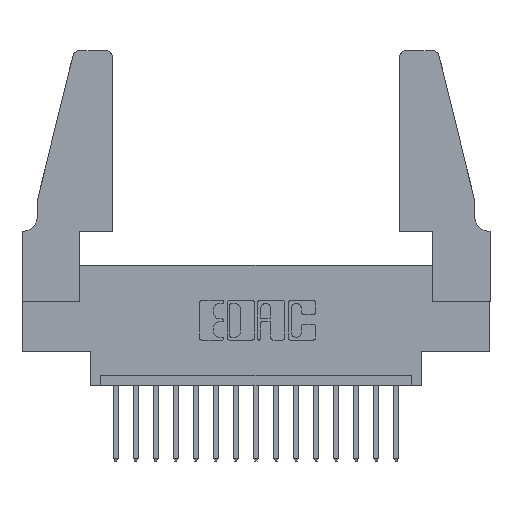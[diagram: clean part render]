
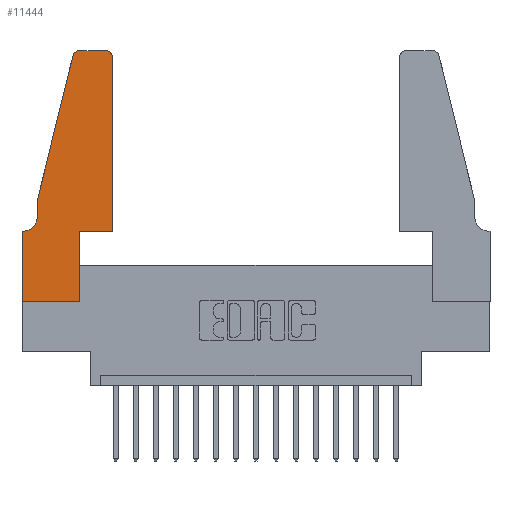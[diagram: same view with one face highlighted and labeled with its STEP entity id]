
A CAD part, top view. The second image highlights one B-rep face of the part: STEP entity #11444.
In plain terms, the highlighted planar face has unit normal (0, 0, 1).
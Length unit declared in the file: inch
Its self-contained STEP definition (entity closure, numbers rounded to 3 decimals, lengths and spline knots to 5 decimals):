
#1 = ORIENTED_EDGE ( 'NONE', *, *, #2793, .T. ) ;
#16 = VERTEX_POINT ( 'NONE', #2848 ) ;
#237 = VERTEX_POINT ( 'NONE', #4636 ) ;
#336 = CARTESIAN_POINT ( 'NONE',  ( 0.2865, 0.35, 0.37 ) ) ;
#346 = CARTESIAN_POINT ( 'NONE',  ( 0., 0.35, 0.37 ) ) ;
#474 = CARTESIAN_POINT ( 'NONE',  ( 0.284, 1.22, 0.37 ) ) ;
#496 = LINE ( 'NONE', #1769, #7144 ) ;
#559 = CIRCLE ( 'NONE', #1673, 0.03 ) ;
#644 = CARTESIAN_POINT ( 'NONE',  ( 0., 0.35, 0.37 ) ) ;
#1037 = EDGE_CURVE ( 'NONE', #14852, #12721, #2362, .T. ) ;
#1673 = AXIS2_PLACEMENT_3D ( 'NONE', #15870, #8903, #3794 ) ;
#1742 = LINE ( 'NONE', #16412, #12845 ) ;
#1769 = CARTESIAN_POINT ( 'NONE',  ( 0.0755, 0.35, 0.37 ) ) ;
#1813 = LINE ( 'NONE', #14876, #9763 ) ;
#1844 = LINE ( 'NONE', #3562, #11256 ) ;
#2362 = LINE ( 'NONE', #8938, #15721 ) ;
#2401 = DIRECTION ( 'NONE',  ( -1., 0., 0. ) ) ;
#2793 = EDGE_CURVE ( 'NONE', #5024, #7057, #559, .T. ) ;
#2848 = CARTESIAN_POINT ( 'NONE',  ( 0.0755, 0.5, 0.37 ) ) ;
#2955 = EDGE_CURVE ( 'NONE', #16, #11109, #14087, .T. ) ;
#2970 = DIRECTION ( 'NONE',  ( 1., 0., 0. ) ) ;
#3046 = ORIENTED_EDGE ( 'NONE', *, *, #9327, .T. ) ;
#3050 = PLANE ( 'NONE',  #17164 ) ;
#3211 = VECTOR ( 'NONE', #15960, 39.37008 ) ;
#3326 = VECTOR ( 'NONE', #5784, 39.37008 ) ;
#3562 = CARTESIAN_POINT ( 'NONE',  ( 0.2605, 1.25, 0.37 ) ) ;
#3794 = DIRECTION ( 'NONE',  ( 1., 0., 0. ) ) ;
#4121 = ORIENTED_EDGE ( 'NONE', *, *, #4985, .T. ) ;
#4129 = CARTESIAN_POINT ( 'NONE',  ( 0.4505, 0.35, 0.37 ) ) ;
#4493 = ORIENTED_EDGE ( 'NONE', *, *, #2955, .T. ) ;
#4636 = CARTESIAN_POINT ( 'NONE',  ( 0.0055, 0.35, 0.37 ) ) ;
#4691 = CARTESIAN_POINT ( 'NONE',  ( 0., 0., 0.37 ) ) ;
#4951 = CARTESIAN_POINT ( 'NONE',  ( 0., 0., 0.37 ) ) ;
#4985 = EDGE_CURVE ( 'NONE', #237, #10996, #496, .T. ) ;
#5024 = VERTEX_POINT ( 'NONE', #11113 ) ;
#5228 = ORIENTED_EDGE ( 'NONE', *, *, #16265, .T. ) ;
#5450 = CIRCLE ( 'NONE', #11662, 0.03 ) ;
#5626 = EDGE_CURVE ( 'NONE', #14051, #8852, #5450, .T. ) ;
#5661 = ORIENTED_EDGE ( 'NONE', *, *, #1037, .T. ) ;
#5784 = DIRECTION ( 'NONE',  ( 0., 1., 0. ) ) ;
#6559 = EDGE_CURVE ( 'NONE', #10996, #14852, #7705, .T. ) ;
#6657 = ORIENTED_EDGE ( 'NONE', *, *, #13461, .T. ) ;
#6762 = LINE ( 'NONE', #4129, #3211 ) ;
#7057 = VERTEX_POINT ( 'NONE', #14147 ) ;
#7144 = VECTOR ( 'NONE', #16198, 39.37008 ) ;
#7190 = EDGE_CURVE ( 'NONE', #7057, #14051, #1844, .T. ) ;
#7452 = EDGE_LOOP ( 'NONE', ( #12930, #11914, #5228, #4493, #10769, #4121, #9770, #5661, #6657, #3046, #15128, #1 ) ) ;
#7705 = LINE ( 'NONE', #4691, #8124 ) ;
#8124 = VECTOR ( 'NONE', #16687, 39.37008 ) ;
#8438 = DIRECTION ( 'NONE',  ( 1., 0., 0. ) ) ;
#8852 = VERTEX_POINT ( 'NONE', #11741 ) ;
#8870 = FACE_OUTER_BOUND ( 'NONE', #7452, .T. ) ;
#8903 = DIRECTION ( 'NONE',  ( 0., 0., 1. ) ) ;
#8938 = CARTESIAN_POINT ( 'NONE',  ( 0., 0., 0.37 ) ) ;
#9327 = EDGE_CURVE ( 'NONE', #11349, #11127, #1813, .T. ) ;
#9740 = AXIS2_PLACEMENT_3D ( 'NONE', #10851, #13863, #16352 ) ;
#9763 = VECTOR ( 'NONE', #2970, 39.37008 ) ;
#9770 = ORIENTED_EDGE ( 'NONE', *, *, #6559, .T. ) ;
#9908 = CIRCLE ( 'NONE', #9740, 0.07 ) ;
#10408 = CARTESIAN_POINT ( 'NONE',  ( 0.0755, 0.5, 0.37 ) ) ;
#10769 = ORIENTED_EDGE ( 'NONE', *, *, #14454, .T. ) ;
#10851 = CARTESIAN_POINT ( 'NONE',  ( 0.0055, 0.42, 0.37 ) ) ;
#10996 = VERTEX_POINT ( 'NONE', #644 ) ;
#11109 = VERTEX_POINT ( 'NONE', #12894 ) ;
#11113 = CARTESIAN_POINT ( 'NONE',  ( 0.4505, 1.22, 0.37 ) ) ;
#11127 = VERTEX_POINT ( 'NONE', #13217 ) ;
#11210 = DIRECTION ( 'NONE',  ( 0., 0., 1. ) ) ;
#11256 = VECTOR ( 'NONE', #2401, 39.37008 ) ;
#11349 = VERTEX_POINT ( 'NONE', #15940 ) ;
#11444 = ADVANCED_FACE ( 'NONE', ( #8870 ), #3050, .T. ) ;
#11662 = AXIS2_PLACEMENT_3D ( 'NONE', #474, #11210, #8438 ) ;
#11681 = DIRECTION ( 'NONE',  ( 0., -1., 0. ) ) ;
#11741 = CARTESIAN_POINT ( 'NONE',  ( 0.25487, 1.22718, 0.37 ) ) ;
#11914 = ORIENTED_EDGE ( 'NONE', *, *, #5626, .T. ) ;
#12289 = DIRECTION ( 'NONE',  ( 1., 0., 0. ) ) ;
#12721 = VERTEX_POINT ( 'NONE', #15077 ) ;
#12845 = VECTOR ( 'NONE', #13798, 39.37008 ) ;
#12894 = CARTESIAN_POINT ( 'NONE',  ( 0.0755, 0.42, 0.37 ) ) ;
#12930 = ORIENTED_EDGE ( 'NONE', *, *, #7190, .T. ) ;
#13217 = CARTESIAN_POINT ( 'NONE',  ( 0.4505, 0.35, 0.37 ) ) ;
#13461 = EDGE_CURVE ( 'NONE', #12721, #11349, #16900, .T. ) ;
#13798 = DIRECTION ( 'NONE',  ( -0.239, -0.971, 0. ) ) ;
#13822 = CARTESIAN_POINT ( 'NONE',  ( 0.284, 1.25, 0.37 ) ) ;
#13863 = DIRECTION ( 'NONE',  ( 0., 0., -1. ) ) ;
#14051 = VERTEX_POINT ( 'NONE', #13822 ) ;
#14087 = LINE ( 'NONE', #10408, #17205 ) ;
#14147 = CARTESIAN_POINT ( 'NONE',  ( 0.4205, 1.25, 0.37 ) ) ;
#14454 = EDGE_CURVE ( 'NONE', #11109, #237, #9908, .T. ) ;
#14852 = VERTEX_POINT ( 'NONE', #4951 ) ;
#14876 = CARTESIAN_POINT ( 'NONE',  ( 0.4505, 0.35, 0.37 ) ) ;
#15010 = DIRECTION ( 'NONE',  ( 1., 0., 0. ) ) ;
#15077 = CARTESIAN_POINT ( 'NONE',  ( 0.2865, 0., 0.37 ) ) ;
#15128 = ORIENTED_EDGE ( 'NONE', *, *, #15610, .T. ) ;
#15610 = EDGE_CURVE ( 'NONE', #11127, #5024, #6762, .T. ) ;
#15721 = VECTOR ( 'NONE', #12289, 39.37008 ) ;
#15870 = CARTESIAN_POINT ( 'NONE',  ( 0.4205, 1.22, 0.37 ) ) ;
#15940 = CARTESIAN_POINT ( 'NONE',  ( 0.2865, 0.35, 0.37 ) ) ;
#15960 = DIRECTION ( 'NONE',  ( 0., 1., 0. ) ) ;
#16198 = DIRECTION ( 'NONE',  ( -1., 0., 0. ) ) ;
#16265 = EDGE_CURVE ( 'NONE', #8852, #16, #1742, .T. ) ;
#16281 = DIRECTION ( 'NONE',  ( 0., 0., 1. ) ) ;
#16352 = DIRECTION ( 'NONE',  ( -1., 0., 0. ) ) ;
#16412 = CARTESIAN_POINT ( 'NONE',  ( 0.0755, 0.5, 0.37 ) ) ;
#16687 = DIRECTION ( 'NONE',  ( 0., -1., 0. ) ) ;
#16900 = LINE ( 'NONE', #336, #3326 ) ;
#17164 = AXIS2_PLACEMENT_3D ( 'NONE', #346, #16281, #15010 ) ;
#17205 = VECTOR ( 'NONE', #11681, 39.37008 ) ;
